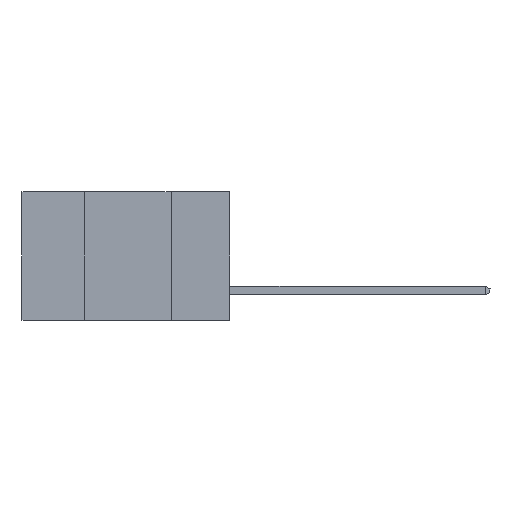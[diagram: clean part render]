
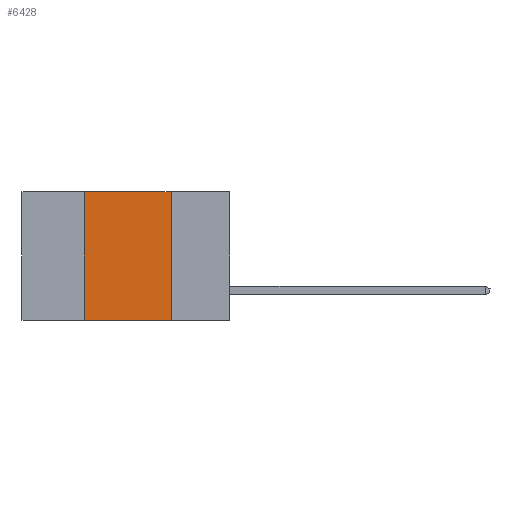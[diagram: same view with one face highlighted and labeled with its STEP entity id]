
A CAD part, left-side view. The second image highlights one B-rep face of the part: STEP entity #6428.
In plain terms, the highlighted planar face has unit normal (-1, 0, 0).
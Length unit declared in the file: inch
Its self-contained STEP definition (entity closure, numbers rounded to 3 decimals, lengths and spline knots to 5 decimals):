
#371 = LINE ( 'NONE', #4097, #6374 ) ;
#384 = VERTEX_POINT ( 'NONE', #7239 ) ;
#417 = EDGE_CURVE ( 'NONE', #8001, #4961, #371, .T. ) ;
#563 = CARTESIAN_POINT ( 'NONE',  ( 0., 0.6, 0. ) ) ;
#954 = ORIENTED_EDGE ( 'NONE', *, *, #1948, .T. ) ;
#1008 = VECTOR ( 'NONE', #5739, 39.37008 ) ;
#1242 = ORIENTED_EDGE ( 'NONE', *, *, #417, .F. ) ;
#1311 = LINE ( 'NONE', #1940, #1008 ) ;
#1340 = LINE ( 'NONE', #6355, #3546 ) ;
#1573 = ORIENTED_EDGE ( 'NONE', *, *, #4593, .F. ) ;
#1588 = VERTEX_POINT ( 'NONE', #3295 ) ;
#1639 = ORIENTED_EDGE ( 'NONE', *, *, #5061, .F. ) ;
#1867 = PLANE ( 'NONE',  #6394 ) ;
#1940 = CARTESIAN_POINT ( 'NONE',  ( 0., 0.17, -0.37 ) ) ;
#1948 = EDGE_CURVE ( 'NONE', #8001, #384, #7607, .T. ) ;
#3024 = FACE_OUTER_BOUND ( 'NONE', #8267, .T. ) ;
#3110 = DIRECTION ( 'NONE',  ( 1., 0., 0. ) ) ;
#3295 = CARTESIAN_POINT ( 'NONE',  ( 0., 0.17, 0. ) ) ;
#3546 = VECTOR ( 'NONE', #7703, 39.37008 ) ;
#4097 = CARTESIAN_POINT ( 'NONE',  ( 0., 0.42, -0.37 ) ) ;
#4174 = DIRECTION ( 'NONE',  ( 0., 0., 1. ) ) ;
#4593 = EDGE_CURVE ( 'NONE', #1588, #384, #1311, .T. ) ;
#4961 = VERTEX_POINT ( 'NONE', #4974 ) ;
#4974 = CARTESIAN_POINT ( 'NONE',  ( 0., 0.42, 0. ) ) ;
#5061 = EDGE_CURVE ( 'NONE', #4961, #1588, #1340, .T. ) ;
#5663 = DIRECTION ( 'NONE',  ( 0., 0., -1. ) ) ;
#5739 = DIRECTION ( 'NONE',  ( 0., 0., -1. ) ) ;
#6071 = VECTOR ( 'NONE', #7649, 39.37008 ) ;
#6355 = CARTESIAN_POINT ( 'NONE',  ( 0., 0.6, 0. ) ) ;
#6374 = VECTOR ( 'NONE', #4174, 39.37008 ) ;
#6394 = AXIS2_PLACEMENT_3D ( 'NONE', #563, #3110, #5663 ) ;
#6428 = ADVANCED_FACE ( 'NONE', ( #3024 ), #1867, .F. ) ;
#6634 = CARTESIAN_POINT ( 'NONE',  ( 0., 0.42, -0.37 ) ) ;
#7239 = CARTESIAN_POINT ( 'NONE',  ( 0., 0.17, -0.37 ) ) ;
#7562 = CARTESIAN_POINT ( 'NONE',  ( 0., 0.6, -0.37 ) ) ;
#7607 = LINE ( 'NONE', #7562, #6071 ) ;
#7649 = DIRECTION ( 'NONE',  ( 0., -1., 0. ) ) ;
#7703 = DIRECTION ( 'NONE',  ( 0., -1., 0. ) ) ;
#8001 = VERTEX_POINT ( 'NONE', #6634 ) ;
#8267 = EDGE_LOOP ( 'NONE', ( #1573, #1639, #1242, #954 ) ) ;
